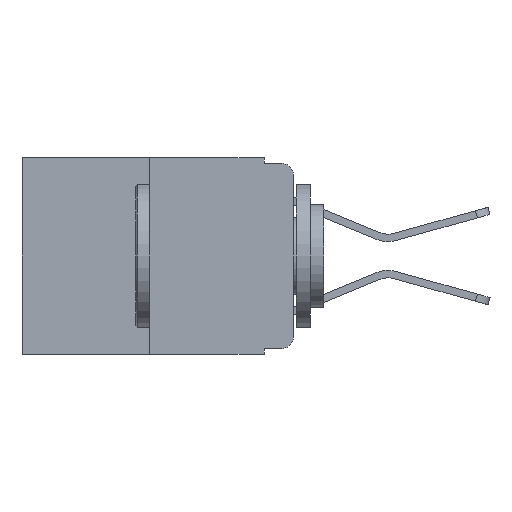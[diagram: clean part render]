
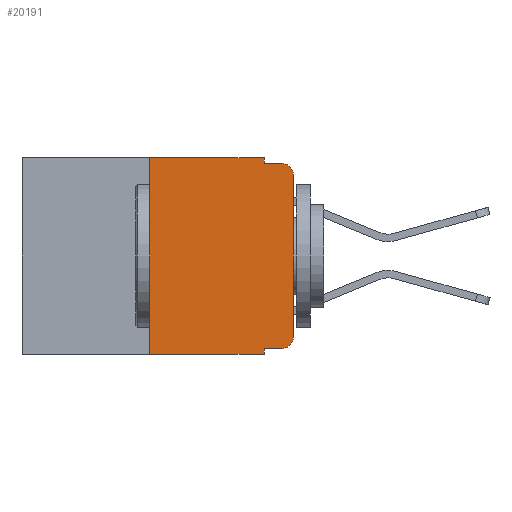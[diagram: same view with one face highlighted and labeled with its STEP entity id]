
A CAD part, left-side view. The second image highlights one B-rep face of the part: STEP entity #20191.
In plain terms, the highlighted planar face has unit normal (-1, 0, 0).
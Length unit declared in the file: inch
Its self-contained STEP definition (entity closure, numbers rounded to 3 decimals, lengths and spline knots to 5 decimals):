
#533 = AXIS2_PLACEMENT_3D ( 'NONE', #17178, #13583, #924 ) ;
#797 = ORIENTED_EDGE ( 'NONE', *, *, #7872, .F. ) ;
#924 = DIRECTION ( 'NONE',  ( 0., 0., -1. ) ) ;
#1319 = CIRCLE ( 'NONE', #9044, 0.02 ) ;
#1519 = VECTOR ( 'NONE', #19297, 39.37008 ) ;
#1695 = CARTESIAN_POINT ( 'NONE',  ( 0., 0.02, -0.03 ) ) ;
#1730 = CARTESIAN_POINT ( 'NONE',  ( 0., 0.473, -0.343 ) ) ;
#1731 = ORIENTED_EDGE ( 'NONE', *, *, #2947, .F. ) ;
#1887 = EDGE_CURVE ( 'NONE', #4999, #20556, #1319, .T. ) ;
#2163 = VERTEX_POINT ( 'NONE', #5935 ) ;
#2805 = ORIENTED_EDGE ( 'NONE', *, *, #17711, .T. ) ;
#2947 = EDGE_CURVE ( 'NONE', #12302, #8055, #17466, .T. ) ;
#3115 = CARTESIAN_POINT ( 'NONE',  ( 0., 0.051, 0. ) ) ;
#3561 = EDGE_CURVE ( 'NONE', #21167, #5018, #3772, .T. ) ;
#3772 = CIRCLE ( 'NONE', #17877, 0.02 ) ;
#4061 = CARTESIAN_POINT ( 'NONE',  ( 0., 0.25, 0. ) ) ;
#4516 = CARTESIAN_POINT ( 'NONE',  ( 0., 0.051, 0. ) ) ;
#4693 = VERTEX_POINT ( 'NONE', #4516 ) ;
#4903 = EDGE_CURVE ( 'NONE', #17945, #20556, #14306, .T. ) ;
#4999 = VERTEX_POINT ( 'NONE', #7685 ) ;
#5018 = VERTEX_POINT ( 'NONE', #11278 ) ;
#5034 = CARTESIAN_POINT ( 'NONE',  ( 0., 0.051, -0.343 ) ) ;
#5498 = VECTOR ( 'NONE', #19457, 39.37008 ) ;
#5935 = CARTESIAN_POINT ( 'NONE',  ( 0., 0.051, -0.333 ) ) ;
#7206 = DIRECTION ( 'NONE',  ( -1., 0., 0. ) ) ;
#7352 = DIRECTION ( 'NONE',  ( 0., 0., -1. ) ) ;
#7502 = FACE_OUTER_BOUND ( 'NONE', #20824, .T. ) ;
#7685 = CARTESIAN_POINT ( 'NONE',  ( 0., 0., -0.03 ) ) ;
#7872 = EDGE_CURVE ( 'NONE', #8055, #4693, #16670, .T. ) ;
#8055 = VERTEX_POINT ( 'NONE', #4061 ) ;
#9044 = AXIS2_PLACEMENT_3D ( 'NONE', #1695, #13327, #10863 ) ;
#9237 = ORIENTED_EDGE ( 'NONE', *, *, #4903, .F. ) ;
#9603 = ORIENTED_EDGE ( 'NONE', *, *, #12283, .T. ) ;
#10066 = CARTESIAN_POINT ( 'NONE',  ( 0., 0.051, -0.333 ) ) ;
#10170 = VECTOR ( 'NONE', #23109, 39.37008 ) ;
#10293 = CARTESIAN_POINT ( 'NONE',  ( 0., 0.051, -0.01 ) ) ;
#10422 = VECTOR ( 'NONE', #20524, 39.37008 ) ;
#10505 = LINE ( 'NONE', #10066, #21412 ) ;
#10863 = DIRECTION ( 'NONE',  ( 0., 0., -1. ) ) ;
#11278 = CARTESIAN_POINT ( 'NONE',  ( 0., 0., -0.313 ) ) ;
#11582 = VECTOR ( 'NONE', #19202, 39.37008 ) ;
#11636 = LINE ( 'NONE', #3115, #1519 ) ;
#12104 = CARTESIAN_POINT ( 'NONE',  ( 0., 0., 0. ) ) ;
#12283 = EDGE_CURVE ( 'NONE', #2163, #21167, #10505, .T. ) ;
#12302 = VERTEX_POINT ( 'NONE', #15587 ) ;
#12540 = ORIENTED_EDGE ( 'NONE', *, *, #1887, .T. ) ;
#13135 = EDGE_CURVE ( 'NONE', #5018, #4999, #21354, .T. ) ;
#13327 = DIRECTION ( 'NONE',  ( -1., 0., 0. ) ) ;
#13583 = DIRECTION ( 'NONE',  ( 1., 0., 0. ) ) ;
#14067 = EDGE_CURVE ( 'NONE', #4693, #17945, #15434, .T. ) ;
#14306 = LINE ( 'NONE', #10293, #22996 ) ;
#14393 = CARTESIAN_POINT ( 'NONE',  ( 0., 0.473, 0. ) ) ;
#14906 = LINE ( 'NONE', #1730, #10170 ) ;
#15276 = DIRECTION ( 'NONE',  ( 0., 0., 1. ) ) ;
#15403 = PLANE ( 'NONE',  #533 ) ;
#15434 = LINE ( 'NONE', #21716, #10422 ) ;
#15587 = CARTESIAN_POINT ( 'NONE',  ( 0., 0.25, -0.343 ) ) ;
#15658 = DIRECTION ( 'NONE',  ( 0., -1., 0. ) ) ;
#16166 = CARTESIAN_POINT ( 'NONE',  ( 0., 0.02, -0.313 ) ) ;
#16323 = ORIENTED_EDGE ( 'NONE', *, *, #3561, .T. ) ;
#16643 = VECTOR ( 'NONE', #15276, 39.37008 ) ;
#16670 = LINE ( 'NONE', #14393, #5498 ) ;
#17178 = CARTESIAN_POINT ( 'NONE',  ( 0., 0.473, 0. ) ) ;
#17466 = LINE ( 'NONE', #18787, #16643 ) ;
#17711 = EDGE_CURVE ( 'NONE', #12302, #19570, #14906, .T. ) ;
#17877 = AXIS2_PLACEMENT_3D ( 'NONE', #16166, #7206, #7352 ) ;
#17945 = VERTEX_POINT ( 'NONE', #18057 ) ;
#18057 = CARTESIAN_POINT ( 'NONE',  ( 0., 0.051, -0.01 ) ) ;
#18298 = ORIENTED_EDGE ( 'NONE', *, *, #21924, .F. ) ;
#18316 = ORIENTED_EDGE ( 'NONE', *, *, #13135, .T. ) ;
#18787 = CARTESIAN_POINT ( 'NONE',  ( 0., 0.25, 0. ) ) ;
#19020 = DIRECTION ( 'NONE',  ( 0., -1., 0. ) ) ;
#19202 = DIRECTION ( 'NONE',  ( 0., 0., 1. ) ) ;
#19297 = DIRECTION ( 'NONE',  ( 0., 0., -1. ) ) ;
#19457 = DIRECTION ( 'NONE',  ( 0., -1., 0. ) ) ;
#19570 = VERTEX_POINT ( 'NONE', #5034 ) ;
#20191 = ADVANCED_FACE ( 'NONE', ( #7502 ), #15403, .F. ) ;
#20193 = CARTESIAN_POINT ( 'NONE',  ( 0., 0.02, -0.333 ) ) ;
#20438 = CARTESIAN_POINT ( 'NONE',  ( 0., 0.02, -0.01 ) ) ;
#20524 = DIRECTION ( 'NONE',  ( 0., 0., -1. ) ) ;
#20556 = VERTEX_POINT ( 'NONE', #20438 ) ;
#20752 = ORIENTED_EDGE ( 'NONE', *, *, #14067, .F. ) ;
#20824 = EDGE_LOOP ( 'NONE', ( #18316, #12540, #9237, #20752, #797, #1731, #2805, #18298, #9603, #16323 ) ) ;
#21167 = VERTEX_POINT ( 'NONE', #20193 ) ;
#21354 = LINE ( 'NONE', #12104, #11582 ) ;
#21412 = VECTOR ( 'NONE', #19020, 39.37008 ) ;
#21716 = CARTESIAN_POINT ( 'NONE',  ( 0., 0.051, 0. ) ) ;
#21924 = EDGE_CURVE ( 'NONE', #2163, #19570, #11636, .T. ) ;
#22996 = VECTOR ( 'NONE', #15658, 39.37008 ) ;
#23109 = DIRECTION ( 'NONE',  ( 0., -1., 0. ) ) ;
